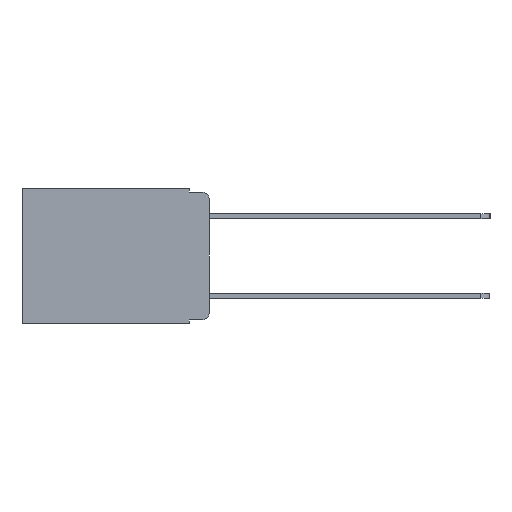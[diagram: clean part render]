
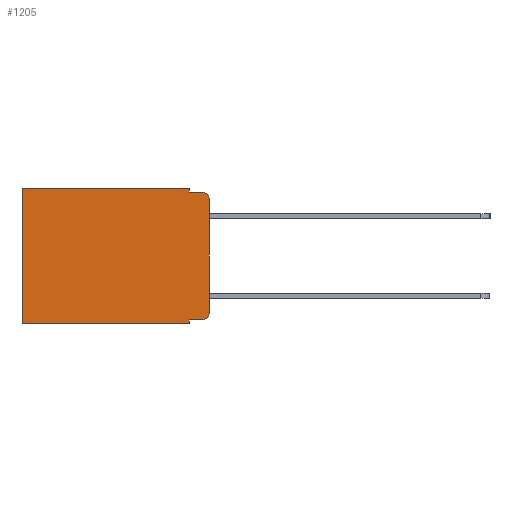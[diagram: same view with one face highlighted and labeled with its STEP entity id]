
A CAD part, left-side view. The second image highlights one B-rep face of the part: STEP entity #1205.
In plain terms, the highlighted planar face has unit normal (-1, 0, 0).
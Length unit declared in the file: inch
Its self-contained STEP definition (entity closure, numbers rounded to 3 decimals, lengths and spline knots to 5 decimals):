
#132 = LINE ( 'NONE', #1324, #8761 ) ;
#365 = LINE ( 'NONE', #1361, #9188 ) ;
#399 = ORIENTED_EDGE ( 'NONE', *, *, #1852, .T. ) ;
#466 = ORIENTED_EDGE ( 'NONE', *, *, #9246, .F. ) ;
#564 = EDGE_CURVE ( 'NONE', #7709, #1243, #5021, .T. ) ;
#692 = VERTEX_POINT ( 'NONE', #1859 ) ;
#736 = VERTEX_POINT ( 'NONE', #10532 ) ;
#738 = LINE ( 'NONE', #2432, #9459 ) ;
#883 = VERTEX_POINT ( 'NONE', #9903 ) ;
#940 = ORIENTED_EDGE ( 'NONE', *, *, #4789, .T. ) ;
#1048 = CARTESIAN_POINT ( 'NONE',  ( 0.298, 0.051, 0. ) ) ;
#1205 = ADVANCED_FACE ( 'NONE', ( #5039 ), #9175, .F. ) ;
#1243 = VERTEX_POINT ( 'NONE', #2317 ) ;
#1324 = CARTESIAN_POINT ( 'NONE',  ( 0.298, 0.051, -0.01 ) ) ;
#1339 = CARTESIAN_POINT ( 'NONE',  ( 0.298, 0.02, -0.333 ) ) ;
#1349 = CARTESIAN_POINT ( 'NONE',  ( 0.298, 0., 0. ) ) ;
#1361 = CARTESIAN_POINT ( 'NONE',  ( 0.298, 0., -0.343 ) ) ;
#1367 = CARTESIAN_POINT ( 'NONE',  ( 0.298, 0.051, 0. ) ) ;
#1684 = ORIENTED_EDGE ( 'NONE', *, *, #2745, .F. ) ;
#1703 = ORIENTED_EDGE ( 'NONE', *, *, #10836, .F. ) ;
#1757 = DIRECTION ( 'NONE',  ( 0., 0., -1. ) ) ;
#1835 = ORIENTED_EDGE ( 'NONE', *, *, #8225, .F. ) ;
#1852 = EDGE_CURVE ( 'NONE', #883, #7046, #5823, .T. ) ;
#1859 = CARTESIAN_POINT ( 'NONE',  ( 0.298, 0.051, -0.01 ) ) ;
#1987 = DIRECTION ( 'NONE',  ( 0., 0., -1. ) ) ;
#2212 = CIRCLE ( 'NONE', #8953, 0.02 ) ;
#2221 = VERTEX_POINT ( 'NONE', #4860 ) ;
#2317 = CARTESIAN_POINT ( 'NONE',  ( 0.298, 0.051, -0.343 ) ) ;
#2352 = DIRECTION ( 'NONE',  ( 0., 0., -1. ) ) ;
#2432 = CARTESIAN_POINT ( 'NONE',  ( 0.298, 0.051, -0.333 ) ) ;
#2745 = EDGE_CURVE ( 'NONE', #8086, #2221, #3693, .T. ) ;
#2778 = EDGE_CURVE ( 'NONE', #7709, #7500, #738, .T. ) ;
#2815 = ORIENTED_EDGE ( 'NONE', *, *, #564, .F. ) ;
#2900 = CARTESIAN_POINT ( 'NONE',  ( 0.298, 0., -0.03 ) ) ;
#3693 = LINE ( 'NONE', #1349, #7908 ) ;
#4024 = AXIS2_PLACEMENT_3D ( 'NONE', #6102, #6091, #6084 ) ;
#4789 = EDGE_CURVE ( 'NONE', #7046, #6912, #9747, .T. ) ;
#4860 = CARTESIAN_POINT ( 'NONE',  ( 0.298, 0., -0.313 ) ) ;
#4873 = ORIENTED_EDGE ( 'NONE', *, *, #5843, .T. ) ;
#5021 = LINE ( 'NONE', #1367, #9136 ) ;
#5024 = DIRECTION ( 'NONE',  ( -1., 0., 0. ) ) ;
#5039 = FACE_OUTER_BOUND ( 'NONE', #10705, .T. ) ;
#5681 = DIRECTION ( 'NONE',  ( 0., 1., 0. ) ) ;
#5823 = LINE ( 'NONE', #10156, #8062 ) ;
#5843 = EDGE_CURVE ( 'NONE', #7500, #2221, #8120, .T. ) ;
#6084 = DIRECTION ( 'NONE',  ( 0., 0., -1. ) ) ;
#6091 = DIRECTION ( 'NONE',  ( -1., 0., 0. ) ) ;
#6102 = CARTESIAN_POINT ( 'NONE',  ( 0.298, 0.02, -0.313 ) ) ;
#6108 = ORIENTED_EDGE ( 'NONE', *, *, #2778, .T. ) ;
#6348 = DIRECTION ( 'NONE',  ( 1., 0., 0. ) ) ;
#6487 = DIRECTION ( 'NONE',  ( 0., 1., 0. ) ) ;
#6808 = CARTESIAN_POINT ( 'NONE',  ( 0.298, 0.473, 0. ) ) ;
#6912 = VERTEX_POINT ( 'NONE', #7520 ) ;
#7046 = VERTEX_POINT ( 'NONE', #6808 ) ;
#7194 = VECTOR ( 'NONE', #9590, 39.37008 ) ;
#7241 = VECTOR ( 'NONE', #1987, 39.37008 ) ;
#7317 = AXIS2_PLACEMENT_3D ( 'NONE', #8781, #6348, #2352 ) ;
#7500 = VERTEX_POINT ( 'NONE', #1339 ) ;
#7520 = CARTESIAN_POINT ( 'NONE',  ( 0.298, 0.473, -0.343 ) ) ;
#7577 = CARTESIAN_POINT ( 'NONE',  ( 0.298, 0.051, -0.333 ) ) ;
#7684 = EDGE_CURVE ( 'NONE', #8086, #736, #2212, .T. ) ;
#7709 = VERTEX_POINT ( 'NONE', #7577 ) ;
#7908 = VECTOR ( 'NONE', #1757, 39.37008 ) ;
#8062 = VECTOR ( 'NONE', #5681, 39.37008 ) ;
#8086 = VERTEX_POINT ( 'NONE', #2900 ) ;
#8120 = CIRCLE ( 'NONE', #4024, 0.02 ) ;
#8152 = DIRECTION ( 'NONE',  ( 0., -1., 0. ) ) ;
#8225 = EDGE_CURVE ( 'NONE', #692, #736, #132, .T. ) ;
#8761 = VECTOR ( 'NONE', #8152, 39.37008 ) ;
#8781 = CARTESIAN_POINT ( 'NONE',  ( 0.298, 0., 0. ) ) ;
#8790 = DIRECTION ( 'NONE',  ( 0., 0., -1. ) ) ;
#8953 = AXIS2_PLACEMENT_3D ( 'NONE', #9846, #5024, #10597 ) ;
#9136 = VECTOR ( 'NONE', #8790, 39.37008 ) ;
#9175 = PLANE ( 'NONE',  #7317 ) ;
#9188 = VECTOR ( 'NONE', #6487, 39.37008 ) ;
#9246 = EDGE_CURVE ( 'NONE', #883, #692, #9556, .T. ) ;
#9459 = VECTOR ( 'NONE', #9857, 39.37008 ) ;
#9556 = LINE ( 'NONE', #1048, #7241 ) ;
#9568 = CARTESIAN_POINT ( 'NONE',  ( 0.298, 0.473, 0. ) ) ;
#9590 = DIRECTION ( 'NONE',  ( 0., 0., -1. ) ) ;
#9694 = ORIENTED_EDGE ( 'NONE', *, *, #7684, .T. ) ;
#9747 = LINE ( 'NONE', #9568, #7194 ) ;
#9846 = CARTESIAN_POINT ( 'NONE',  ( 0.298, 0.02, -0.03 ) ) ;
#9857 = DIRECTION ( 'NONE',  ( 0., -1., 0. ) ) ;
#9903 = CARTESIAN_POINT ( 'NONE',  ( 0.298, 0.051, 0. ) ) ;
#10156 = CARTESIAN_POINT ( 'NONE',  ( 0.298, 0., 0. ) ) ;
#10532 = CARTESIAN_POINT ( 'NONE',  ( 0.298, 0.02, -0.01 ) ) ;
#10597 = DIRECTION ( 'NONE',  ( 0., 0., -1. ) ) ;
#10705 = EDGE_LOOP ( 'NONE', ( #1684, #9694, #1835, #466, #399, #940, #1703, #2815, #6108, #4873 ) ) ;
#10836 = EDGE_CURVE ( 'NONE', #1243, #6912, #365, .T. ) ;
